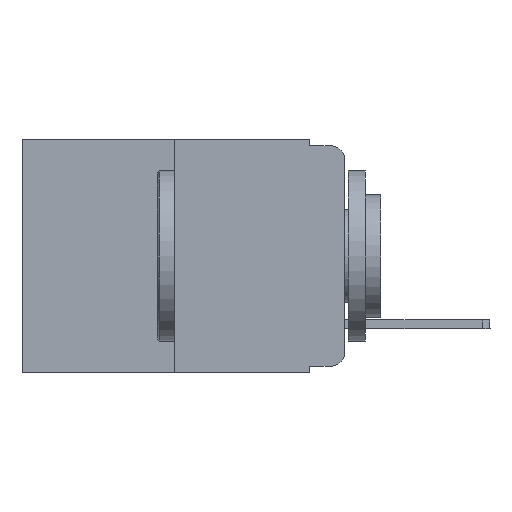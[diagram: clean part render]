
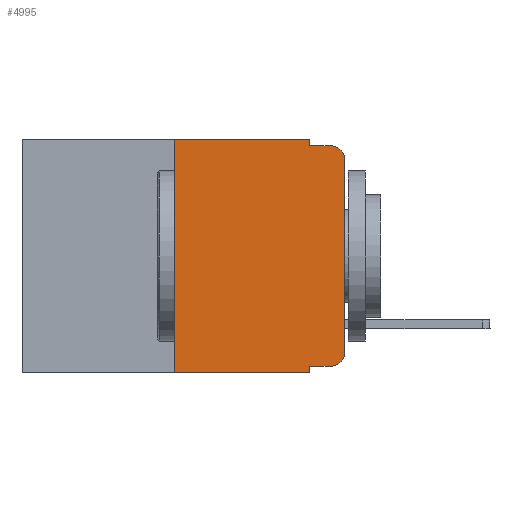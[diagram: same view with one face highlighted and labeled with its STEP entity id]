
A CAD part, left-side view. The second image highlights one B-rep face of the part: STEP entity #4995.
In plain terms, the highlighted planar face has unit normal (-1, 0, 0).
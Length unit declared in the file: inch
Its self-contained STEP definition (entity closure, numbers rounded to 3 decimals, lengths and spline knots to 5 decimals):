
#10 = AXIS2_PLACEMENT_3D ( 'NONE', #11096, #3504, #12378 ) ;
#358 = LINE ( 'NONE', #12443, #549 ) ;
#508 = EDGE_CURVE ( 'NONE', #11054, #8826, #9590, .T. ) ;
#533 = DIRECTION ( 'NONE',  ( 0., 0., -1. ) ) ;
#549 = VECTOR ( 'NONE', #6100, 39.37008 ) ;
#705 = CARTESIAN_POINT ( 'NONE',  ( 0., 0.02, -0.333 ) ) ;
#711 = VERTEX_POINT ( 'NONE', #3190 ) ;
#919 = FACE_OUTER_BOUND ( 'NONE', #14850, .T. ) ;
#1082 = ORIENTED_EDGE ( 'NONE', *, *, #10878, .F. ) ;
#1179 = EDGE_CURVE ( 'NONE', #16500, #8826, #3826, .T. ) ;
#1379 = DIRECTION ( 'NONE',  ( 0., 0., 1. ) ) ;
#1845 = VERTEX_POINT ( 'NONE', #9164 ) ;
#1878 = CIRCLE ( 'NONE', #15877, 0.02 ) ;
#1885 = CARTESIAN_POINT ( 'NONE',  ( 0., 0.051, 0. ) ) ;
#2007 = EDGE_CURVE ( 'NONE', #11054, #9668, #12126, .T. ) ;
#2638 = VECTOR ( 'NONE', #9413, 39.37008 ) ;
#2952 = ORIENTED_EDGE ( 'NONE', *, *, #2007, .F. ) ;
#2976 = EDGE_CURVE ( 'NONE', #16500, #12114, #358, .T. ) ;
#3102 = DIRECTION ( 'NONE',  ( 0., 0., -1. ) ) ;
#3190 = CARTESIAN_POINT ( 'NONE',  ( 0., 0., -0.313 ) ) ;
#3274 = CARTESIAN_POINT ( 'NONE',  ( 0., 0.473, 0. ) ) ;
#3504 = DIRECTION ( 'NONE',  ( -1., 0., 0. ) ) ;
#3826 = LINE ( 'NONE', #1885, #16131 ) ;
#3872 = CARTESIAN_POINT ( 'NONE',  ( 0., 0.02, -0.313 ) ) ;
#4079 = AXIS2_PLACEMENT_3D ( 'NONE', #5621, #7025, #12024 ) ;
#4239 = ORIENTED_EDGE ( 'NONE', *, *, #5224, .F. ) ;
#4263 = ORIENTED_EDGE ( 'NONE', *, *, #1179, .F. ) ;
#4360 = ORIENTED_EDGE ( 'NONE', *, *, #5869, .T. ) ;
#4539 = DIRECTION ( 'NONE',  ( 0., -1., 0. ) ) ;
#4633 = CARTESIAN_POINT ( 'NONE',  ( 0., 0.25, 0. ) ) ;
#4995 = ADVANCED_FACE ( 'NONE', ( #919 ), #13290, .F. ) ;
#5154 = CARTESIAN_POINT ( 'NONE',  ( 0., 0., 0. ) ) ;
#5224 = EDGE_CURVE ( 'NONE', #13191, #7203, #9066, .T. ) ;
#5360 = VECTOR ( 'NONE', #15769, 39.37008 ) ;
#5621 = CARTESIAN_POINT ( 'NONE',  ( 0., 0.473, 0. ) ) ;
#5869 = EDGE_CURVE ( 'NONE', #12114, #711, #1878, .T. ) ;
#6100 = DIRECTION ( 'NONE',  ( 0., -1., 0. ) ) ;
#6336 = DIRECTION ( 'NONE',  ( 0., -1., 0. ) ) ;
#6569 = CARTESIAN_POINT ( 'NONE',  ( 0., 0.051, -0.333 ) ) ;
#6655 = CARTESIAN_POINT ( 'NONE',  ( 0., 0.25, -0.343 ) ) ;
#7025 = DIRECTION ( 'NONE',  ( 1., 0., 0. ) ) ;
#7160 = EDGE_CURVE ( 'NONE', #711, #14413, #16358, .T. ) ;
#7203 = VERTEX_POINT ( 'NONE', #10279 ) ;
#7241 = ORIENTED_EDGE ( 'NONE', *, *, #508, .T. ) ;
#8100 = CARTESIAN_POINT ( 'NONE',  ( 0., 0.051, -0.01 ) ) ;
#8826 = VERTEX_POINT ( 'NONE', #13942 ) ;
#9010 = VECTOR ( 'NONE', #4539, 39.37008 ) ;
#9066 = LINE ( 'NONE', #14900, #15615 ) ;
#9164 = CARTESIAN_POINT ( 'NONE',  ( 0., 0.051, 0. ) ) ;
#9413 = DIRECTION ( 'NONE',  ( 0., -1., 0. ) ) ;
#9416 = ORIENTED_EDGE ( 'NONE', *, *, #11993, .F. ) ;
#9590 = LINE ( 'NONE', #15623, #2638 ) ;
#9668 = VERTEX_POINT ( 'NONE', #4633 ) ;
#9816 = LINE ( 'NONE', #3274, #9010 ) ;
#10279 = CARTESIAN_POINT ( 'NONE',  ( 0., 0.02, -0.01 ) ) ;
#10878 = EDGE_CURVE ( 'NONE', #9668, #1845, #9816, .T. ) ;
#11054 = VERTEX_POINT ( 'NONE', #6655 ) ;
#11096 = CARTESIAN_POINT ( 'NONE',  ( 0., 0.02, -0.03 ) ) ;
#11796 = VECTOR ( 'NONE', #533, 39.37008 ) ;
#11993 = EDGE_CURVE ( 'NONE', #1845, #13191, #14356, .T. ) ;
#12024 = DIRECTION ( 'NONE',  ( 0., 0., -1. ) ) ;
#12067 = ORIENTED_EDGE ( 'NONE', *, *, #13446, .T. ) ;
#12114 = VERTEX_POINT ( 'NONE', #705 ) ;
#12126 = LINE ( 'NONE', #14540, #5360 ) ;
#12378 = DIRECTION ( 'NONE',  ( 0., 0., -1. ) ) ;
#12443 = CARTESIAN_POINT ( 'NONE',  ( 0., 0.051, -0.333 ) ) ;
#12748 = DIRECTION ( 'NONE',  ( 0., 0., -1. ) ) ;
#12791 = VECTOR ( 'NONE', #1379, 39.37008 ) ;
#13191 = VERTEX_POINT ( 'NONE', #8100 ) ;
#13290 = PLANE ( 'NONE',  #4079 ) ;
#13446 = EDGE_CURVE ( 'NONE', #14413, #7203, #14295, .T. ) ;
#13942 = CARTESIAN_POINT ( 'NONE',  ( 0., 0.051, -0.343 ) ) ;
#14232 = DIRECTION ( 'NONE',  ( -1., 0., 0. ) ) ;
#14295 = CIRCLE ( 'NONE', #10, 0.02 ) ;
#14356 = LINE ( 'NONE', #15777, #11796 ) ;
#14413 = VERTEX_POINT ( 'NONE', #15426 ) ;
#14433 = ORIENTED_EDGE ( 'NONE', *, *, #7160, .T. ) ;
#14540 = CARTESIAN_POINT ( 'NONE',  ( 0., 0.25, 0. ) ) ;
#14850 = EDGE_LOOP ( 'NONE', ( #14433, #12067, #4239, #9416, #1082, #2952, #7241, #4263, #15226, #4360 ) ) ;
#14900 = CARTESIAN_POINT ( 'NONE',  ( 0., 0.051, -0.01 ) ) ;
#15226 = ORIENTED_EDGE ( 'NONE', *, *, #2976, .T. ) ;
#15426 = CARTESIAN_POINT ( 'NONE',  ( 0., 0., -0.03 ) ) ;
#15615 = VECTOR ( 'NONE', #6336, 39.37008 ) ;
#15623 = CARTESIAN_POINT ( 'NONE',  ( 0., 0.473, -0.343 ) ) ;
#15769 = DIRECTION ( 'NONE',  ( 0., 0., 1. ) ) ;
#15777 = CARTESIAN_POINT ( 'NONE',  ( 0., 0.051, 0. ) ) ;
#15877 = AXIS2_PLACEMENT_3D ( 'NONE', #3872, #14232, #12748 ) ;
#16131 = VECTOR ( 'NONE', #3102, 39.37008 ) ;
#16358 = LINE ( 'NONE', #5154, #12791 ) ;
#16500 = VERTEX_POINT ( 'NONE', #6569 ) ;
